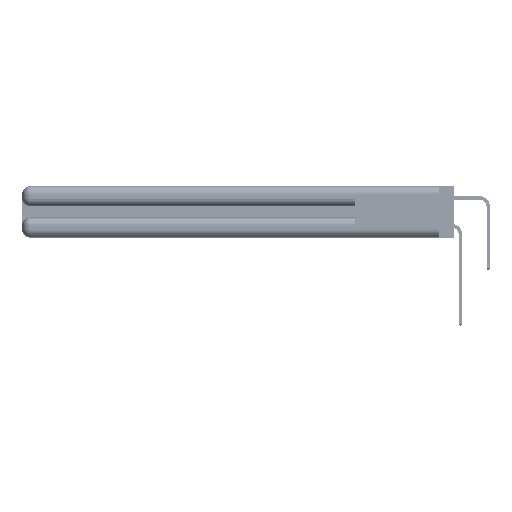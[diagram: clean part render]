
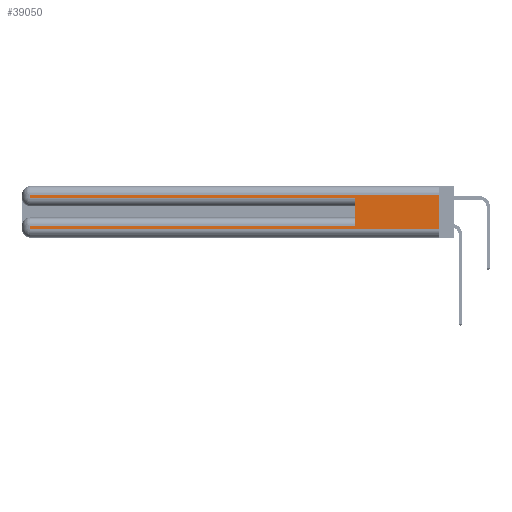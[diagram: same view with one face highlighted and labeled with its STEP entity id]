
A CAD part, left-side view. The second image highlights one B-rep face of the part: STEP entity #39050.
In plain terms, the highlighted planar face has unit normal (-1, 0, 0).
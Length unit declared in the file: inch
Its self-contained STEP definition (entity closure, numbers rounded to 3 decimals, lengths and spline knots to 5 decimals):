
#1337 = CARTESIAN_POINT ( 'NONE',  ( 0., 0., 0.37 ) ) ;
#1514 = PLANE ( 'NONE',  #1698 ) ;
#1698 = AXIS2_PLACEMENT_3D ( 'NONE', #1337, #49424, #25480 ) ;
#2114 = VECTOR ( 'NONE', #28124, 39.37008 ) ;
#2711 = VECTOR ( 'NONE', #40360, 39.37008 ) ;
#3231 = VERTEX_POINT ( 'NONE', #17195 ) ;
#3676 = CARTESIAN_POINT ( 'NONE',  ( 0., 0., 0.285 ) ) ;
#5465 = ORIENTED_EDGE ( 'NONE', *, *, #16016, .T. ) ;
#5495 = EDGE_CURVE ( 'NONE', #3231, #27903, #17481, .T. ) ;
#8145 = VECTOR ( 'NONE', #31639, 39.37008 ) ;
#9231 = VECTOR ( 'NONE', #33755, 39.37008 ) ;
#11153 = EDGE_CURVE ( 'NONE', #43824, #17878, #34715, .T. ) ;
#11805 = CARTESIAN_POINT ( 'NONE',  ( 0., 0., 0.06 ) ) ;
#14330 = ORIENTED_EDGE ( 'NONE', *, *, #40411, .T. ) ;
#14939 = LINE ( 'NONE', #36963, #37370 ) ;
#16016 = EDGE_CURVE ( 'NONE', #20690, #17878, #51030, .T. ) ;
#17195 = CARTESIAN_POINT ( 'NONE',  ( 0., 2.94, 0.085 ) ) ;
#17197 = EDGE_CURVE ( 'NONE', #27903, #45249, #35530, .T. ) ;
#17481 = LINE ( 'NONE', #32384, #24896 ) ;
#17878 = VERTEX_POINT ( 'NONE', #20043 ) ;
#19107 = VECTOR ( 'NONE', #39521, 39.37008 ) ;
#20039 = ORIENTED_EDGE ( 'NONE', *, *, #33851, .T. ) ;
#20043 = CARTESIAN_POINT ( 'NONE',  ( 0., 0.6, 0.285 ) ) ;
#20618 = CARTESIAN_POINT ( 'NONE',  ( 0., 2.94, 0.37 ) ) ;
#20690 = VERTEX_POINT ( 'NONE', #27168 ) ;
#21153 = CARTESIAN_POINT ( 'NONE',  ( 0., 2.94, 0.31 ) ) ;
#23968 = DIRECTION ( 'NONE',  ( 0., 0., -1. ) ) ;
#24055 = VECTOR ( 'NONE', #45811, 39.37008 ) ;
#24896 = VECTOR ( 'NONE', #23968, 39.37008 ) ;
#25480 = DIRECTION ( 'NONE',  ( 0., 0., -1. ) ) ;
#26208 = CARTESIAN_POINT ( 'NONE',  ( 0., 0., 0.085 ) ) ;
#26969 = LINE ( 'NONE', #20618, #2114 ) ;
#27168 = CARTESIAN_POINT ( 'NONE',  ( 0., 2.94, 0.285 ) ) ;
#27903 = VERTEX_POINT ( 'NONE', #34204 ) ;
#28124 = DIRECTION ( 'NONE',  ( 0., 0., -1. ) ) ;
#28394 = DIRECTION ( 'NONE',  ( 0., 0., -1. ) ) ;
#28611 = CARTESIAN_POINT ( 'NONE',  ( 0., 0., 0.31 ) ) ;
#30838 = ORIENTED_EDGE ( 'NONE', *, *, #39546, .F. ) ;
#31639 = DIRECTION ( 'NONE',  ( 0., -1., 0. ) ) ;
#32384 = CARTESIAN_POINT ( 'NONE',  ( 0., 2.94, 0.37 ) ) ;
#33493 = EDGE_LOOP ( 'NONE', ( #30838, #38276, #20039, #5465, #38341, #14330, #34859, #44313 ) ) ;
#33755 = DIRECTION ( 'NONE',  ( 0., 1., 0. ) ) ;
#33851 = EDGE_CURVE ( 'NONE', #36290, #20690, #26969, .T. ) ;
#34204 = CARTESIAN_POINT ( 'NONE',  ( 0., 2.94, 0.06 ) ) ;
#34715 = LINE ( 'NONE', #41449, #24055 ) ;
#34859 = ORIENTED_EDGE ( 'NONE', *, *, #5495, .T. ) ;
#35530 = LINE ( 'NONE', #43520, #8145 ) ;
#36290 = VERTEX_POINT ( 'NONE', #21153 ) ;
#36792 = VERTEX_POINT ( 'NONE', #28611 ) ;
#36963 = CARTESIAN_POINT ( 'NONE',  ( 0., 0., 0.37 ) ) ;
#37370 = VECTOR ( 'NONE', #28394, 39.37008 ) ;
#38276 = ORIENTED_EDGE ( 'NONE', *, *, #42336, .T. ) ;
#38341 = ORIENTED_EDGE ( 'NONE', *, *, #11153, .F. ) ;
#39050 = ADVANCED_FACE ( 'NONE', ( #40514 ), #1514, .F. ) ;
#39521 = DIRECTION ( 'NONE',  ( 0., -1., 0. ) ) ;
#39546 = EDGE_CURVE ( 'NONE', #36792, #45249, #14939, .T. ) ;
#40360 = DIRECTION ( 'NONE',  ( 0., 1., 0. ) ) ;
#40411 = EDGE_CURVE ( 'NONE', #43824, #3231, #49153, .T. ) ;
#40514 = FACE_OUTER_BOUND ( 'NONE', #33493, .T. ) ;
#41449 = CARTESIAN_POINT ( 'NONE',  ( 0., 0.6, 0.145 ) ) ;
#41940 = LINE ( 'NONE', #51562, #2711 ) ;
#42336 = EDGE_CURVE ( 'NONE', #36792, #36290, #41940, .T. ) ;
#43520 = CARTESIAN_POINT ( 'NONE',  ( 0., 0., 0.06 ) ) ;
#43824 = VERTEX_POINT ( 'NONE', #49322 ) ;
#44313 = ORIENTED_EDGE ( 'NONE', *, *, #17197, .T. ) ;
#45249 = VERTEX_POINT ( 'NONE', #11805 ) ;
#45811 = DIRECTION ( 'NONE',  ( 0., 0., 1. ) ) ;
#49153 = LINE ( 'NONE', #26208, #9231 ) ;
#49322 = CARTESIAN_POINT ( 'NONE',  ( 0., 0.6, 0.085 ) ) ;
#49424 = DIRECTION ( 'NONE',  ( 1., 0., 0. ) ) ;
#51030 = LINE ( 'NONE', #3676, #19107 ) ;
#51562 = CARTESIAN_POINT ( 'NONE',  ( 0., 0., 0.31 ) ) ;
